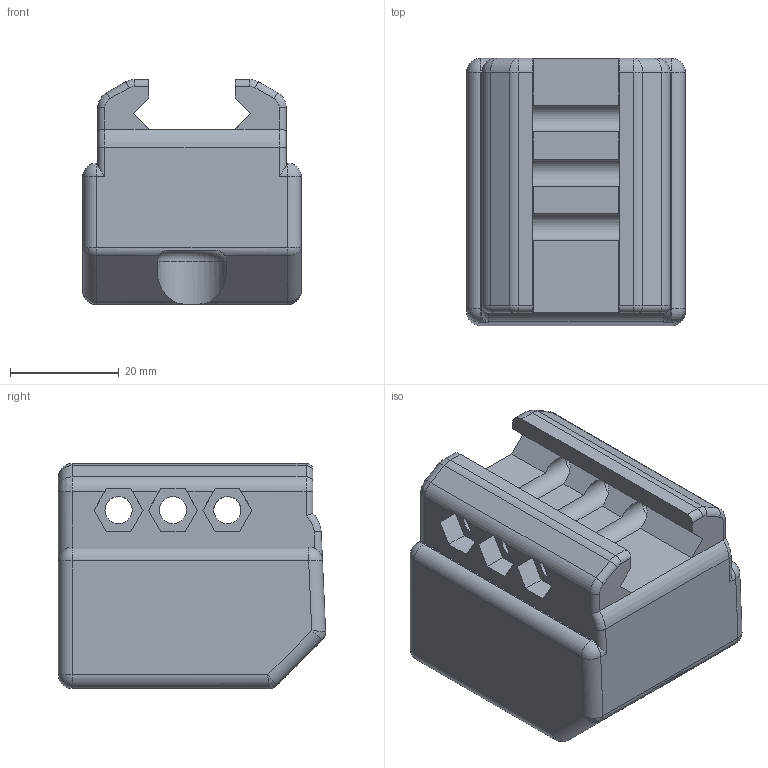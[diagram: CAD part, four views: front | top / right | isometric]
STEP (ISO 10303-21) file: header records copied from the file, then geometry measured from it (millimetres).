
FILE_DESCRIPTION(/* description */ (''),/* implementation_level */ '2;1');
FILE_NAME(/* name */ 'AR15 Buffer Tube Pic Rail Mount.stp',/* time_stamp */ '2021-11-22T21:36:15-06:00',/* author */ ('johne'),/* organization */ (''),/* preprocessor_version */ 'ST-DEVELOPER v18.1',/* originating_system */ 'Autodesk Inventor 2020',/* authorisation */ '');
FILE_SCHEMA (('AUTOMOTIVE_DESIGN { 1 0 10303 214 3 1 1 }'));
Length unit declared in the file: inch
Products named in the file (1): AR15 Buffer Tube Pic Rail Mount
Bounding box: 40.2 x 49.14 x 41.39 mm (x, y, z)
Volume: 50946.8 mm3; surface area: 14686.2 mm2
Topology: 1 solids, 1 shells, 142 faces, 385 edges, 236 vertices
Faces by surface type: plane 61, cylinder 55, bspline 12, torus 7, sphere 6, cone 1
Full cylindrical faces by diameter (mm): 5 x3, 7.3 x3, 29.554 x8
Entity records: 13333 total; most frequent: CARTESIAN_POINT 9741, ORIENTED_EDGE 766, DIRECTION 729, EDGE_CURVE 383, AXIS2_PLACEMENT_3D 261, VERTEX_POINT 238, LINE 207, VECTOR 207
